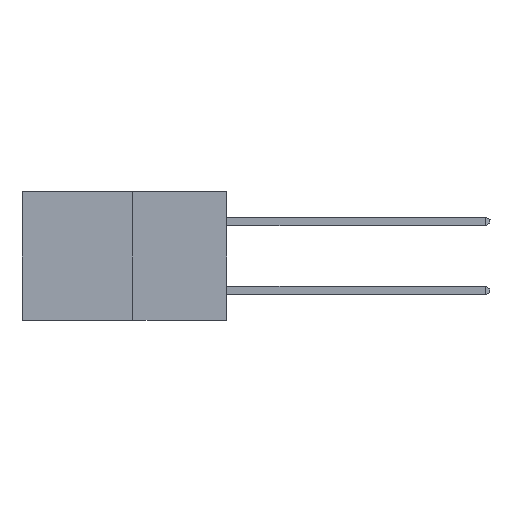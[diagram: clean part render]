
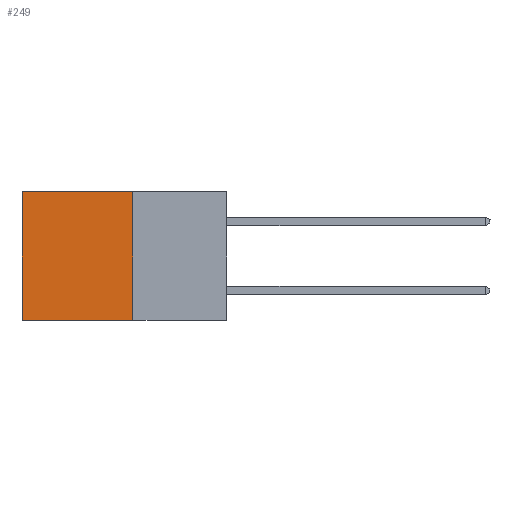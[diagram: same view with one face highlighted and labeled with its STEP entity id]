
A CAD part, left-side view. The second image highlights one B-rep face of the part: STEP entity #249.
In plain terms, the highlighted planar face has unit normal (-1, 0, 0).
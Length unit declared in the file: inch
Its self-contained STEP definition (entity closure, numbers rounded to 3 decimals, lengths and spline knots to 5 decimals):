
#249 = ADVANCED_FACE ( 'NONE', ( #13602 ), #21757, .F. ) ;
#2353 = ORIENTED_EDGE ( 'NONE', *, *, #21772, .T. ) ;
#3072 = CARTESIAN_POINT ( 'NONE',  ( 0.277, 0.27, -0.37 ) ) ;
#3170 = DIRECTION ( 'NONE',  ( 0., 1., 0. ) ) ;
#3910 = VECTOR ( 'NONE', #12546, 39.37008 ) ;
#5244 = CARTESIAN_POINT ( 'NONE',  ( 0.277, 0.27, -0.37 ) ) ;
#5416 = DIRECTION ( 'NONE',  ( 0., 0., -1. ) ) ;
#6606 = EDGE_LOOP ( 'NONE', ( #2353, #13876, #19898, #25433 ) ) ;
#7539 = VECTOR ( 'NONE', #5416, 39.37008 ) ;
#8040 = AXIS2_PLACEMENT_3D ( 'NONE', #3072, #18942, #23815 ) ;
#9267 = DIRECTION ( 'NONE',  ( 0., 0., -1. ) ) ;
#10003 = LINE ( 'NONE', #24414, #3910 ) ;
#11365 = EDGE_CURVE ( 'NONE', #17162, #24382, #20374, .T. ) ;
#11413 = EDGE_CURVE ( 'NONE', #25666, #17162, #13057, .T. ) ;
#12546 = DIRECTION ( 'NONE',  ( 0., 1., 0. ) ) ;
#13057 = LINE ( 'NONE', #17661, #7539 ) ;
#13306 = CARTESIAN_POINT ( 'NONE',  ( 0.277, 0.27, -0.37 ) ) ;
#13602 = FACE_OUTER_BOUND ( 'NONE', #6606, .T. ) ;
#13876 = ORIENTED_EDGE ( 'NONE', *, *, #11365, .F. ) ;
#15284 = CARTESIAN_POINT ( 'NONE',  ( 0.277, 0.59, -0.37 ) ) ;
#15315 = EDGE_CURVE ( 'NONE', #25666, #19782, #10003, .T. ) ;
#17162 = VERTEX_POINT ( 'NONE', #13306 ) ;
#17447 = CARTESIAN_POINT ( 'NONE',  ( 0.277, 0.27, 0. ) ) ;
#17661 = CARTESIAN_POINT ( 'NONE',  ( 0.277, 0.27, -0.37 ) ) ;
#17833 = CARTESIAN_POINT ( 'NONE',  ( 0.277, 0.59, 0. ) ) ;
#18378 = VECTOR ( 'NONE', #9267, 39.37008 ) ;
#18942 = DIRECTION ( 'NONE',  ( 1., 0., 0. ) ) ;
#19012 = LINE ( 'NONE', #19517, #18378 ) ;
#19517 = CARTESIAN_POINT ( 'NONE',  ( 0.277, 0.59, -0.37 ) ) ;
#19774 = VECTOR ( 'NONE', #3170, 39.37008 ) ;
#19782 = VERTEX_POINT ( 'NONE', #17833 ) ;
#19898 = ORIENTED_EDGE ( 'NONE', *, *, #11413, .F. ) ;
#20374 = LINE ( 'NONE', #5244, #19774 ) ;
#21757 = PLANE ( 'NONE',  #8040 ) ;
#21772 = EDGE_CURVE ( 'NONE', #19782, #24382, #19012, .T. ) ;
#23815 = DIRECTION ( 'NONE',  ( 0., 0., -1. ) ) ;
#24382 = VERTEX_POINT ( 'NONE', #15284 ) ;
#24414 = CARTESIAN_POINT ( 'NONE',  ( 0.277, 0.27, 0. ) ) ;
#25433 = ORIENTED_EDGE ( 'NONE', *, *, #15315, .T. ) ;
#25666 = VERTEX_POINT ( 'NONE', #17447 ) ;
